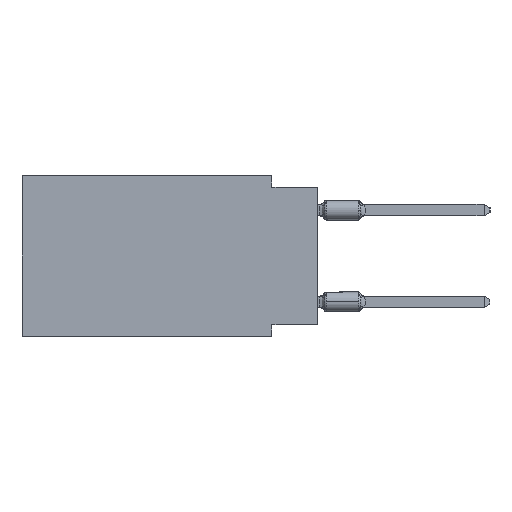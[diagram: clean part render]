
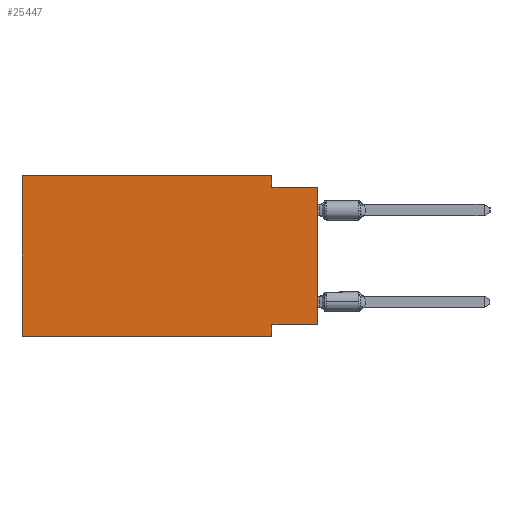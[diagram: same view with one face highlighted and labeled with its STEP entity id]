
A CAD part, left-side view. The second image highlights one B-rep face of the part: STEP entity #25447.
In plain terms, the highlighted planar face has unit normal (-1, 0, 0).
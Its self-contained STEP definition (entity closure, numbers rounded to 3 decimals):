
#44 = ORIENTED_EDGE ( 'NONE', *, *, #25093, .F. ) ;
#259 = LINE ( 'NONE', #33148, #37497 ) ;
#1192 = CARTESIAN_POINT ( 'NONE',  ( 0., 16.383, 0. ) ) ;
#1637 = VERTEX_POINT ( 'NONE', #36387 ) ;
#1899 = ORIENTED_EDGE ( 'NONE', *, *, #34662, .F. ) ;
#2124 = VERTEX_POINT ( 'NONE', #25669 ) ;
#2669 = ORIENTED_EDGE ( 'NONE', *, *, #28378, .F. ) ;
#2726 = VECTOR ( 'NONE', #9663, 1000. ) ;
#3540 = EDGE_CURVE ( 'NONE', #17082, #28157, #30162, .T. ) ;
#4827 = CARTESIAN_POINT ( 'NONE',  ( 0., 0., -8.255 ) ) ;
#5383 = VECTOR ( 'NONE', #29229, 1000. ) ;
#6342 = CARTESIAN_POINT ( 'NONE',  ( 0., 16.383, -8.89 ) ) ;
#7986 = DIRECTION ( 'NONE',  ( 0., 0., 1. ) ) ;
#9663 = DIRECTION ( 'NONE',  ( 0., -1., 0. ) ) ;
#9756 = ORIENTED_EDGE ( 'NONE', *, *, #12859, .F. ) ;
#10096 = CARTESIAN_POINT ( 'NONE',  ( 0., 0., -0.635 ) ) ;
#10932 = CARTESIAN_POINT ( 'NONE',  ( 0., 0., 0. ) ) ;
#10944 = VECTOR ( 'NONE', #24261, 1000. ) ;
#11020 = VERTEX_POINT ( 'NONE', #4827 ) ;
#12067 = LINE ( 'NONE', #21149, #21219 ) ;
#12614 = LINE ( 'NONE', #24622, #2726 ) ;
#12859 = EDGE_CURVE ( 'NONE', #11020, #26576, #22735, .T. ) ;
#13801 = VECTOR ( 'NONE', #31542, 1000. ) ;
#14263 = EDGE_CURVE ( 'NONE', #26576, #28157, #259, .T. ) ;
#16098 = PLANE ( 'NONE',  #33561 ) ;
#16342 = LINE ( 'NONE', #1192, #35155 ) ;
#16647 = EDGE_CURVE ( 'NONE', #11020, #26169, #37870, .T. ) ;
#17082 = VERTEX_POINT ( 'NONE', #27982 ) ;
#17401 = CARTESIAN_POINT ( 'NONE',  ( 0., 0., -8.255 ) ) ;
#19551 = LINE ( 'NONE', #10096, #13801 ) ;
#21149 = CARTESIAN_POINT ( 'NONE',  ( 0., 2.54, 0. ) ) ;
#21219 = VECTOR ( 'NONE', #27449, 1000. ) ;
#21431 = ORIENTED_EDGE ( 'NONE', *, *, #31875, .F. ) ;
#22735 = LINE ( 'NONE', #17401, #5383 ) ;
#24261 = DIRECTION ( 'NONE',  ( 0., -1., 0. ) ) ;
#24622 = CARTESIAN_POINT ( 'NONE',  ( 0., 16.383, 0. ) ) ;
#24906 = ORIENTED_EDGE ( 'NONE', *, *, #16647, .T. ) ;
#25093 = EDGE_CURVE ( 'NONE', #28184, #1637, #12614, .T. ) ;
#25159 = DIRECTION ( 'NONE',  ( 1., 0., 0. ) ) ;
#25247 = EDGE_LOOP ( 'NONE', ( #24906, #1899, #2669, #44, #21431, #28178, #38400, #9756 ) ) ;
#25447 = ADVANCED_FACE ( 'NONE', ( #36555 ), #16098, .F. ) ;
#25669 = CARTESIAN_POINT ( 'NONE',  ( 0., 2.54, -0.635 ) ) ;
#26169 = VERTEX_POINT ( 'NONE', #37380 ) ;
#26576 = VERTEX_POINT ( 'NONE', #27744 ) ;
#27449 = DIRECTION ( 'NONE',  ( 0., 0., -1. ) ) ;
#27744 = CARTESIAN_POINT ( 'NONE',  ( 0., 2.54, -8.255 ) ) ;
#27982 = CARTESIAN_POINT ( 'NONE',  ( 0., 16.383, -8.89 ) ) ;
#28129 = CARTESIAN_POINT ( 'NONE',  ( 0., 16.383, 0. ) ) ;
#28157 = VERTEX_POINT ( 'NONE', #35104 ) ;
#28178 = ORIENTED_EDGE ( 'NONE', *, *, #3540, .T. ) ;
#28184 = VERTEX_POINT ( 'NONE', #34911 ) ;
#28378 = EDGE_CURVE ( 'NONE', #1637, #2124, #12067, .T. ) ;
#29229 = DIRECTION ( 'NONE',  ( 0., 1., 0. ) ) ;
#30162 = LINE ( 'NONE', #6342, #10944 ) ;
#30912 = VECTOR ( 'NONE', #7986, 1000. ) ;
#31542 = DIRECTION ( 'NONE',  ( 0., -1., 0. ) ) ;
#31875 = EDGE_CURVE ( 'NONE', #17082, #28184, #16342, .T. ) ;
#33148 = CARTESIAN_POINT ( 'NONE',  ( 0., 2.54, -8.89 ) ) ;
#33561 = AXIS2_PLACEMENT_3D ( 'NONE', #28129, #25159, #37121 ) ;
#34052 = DIRECTION ( 'NONE',  ( 0., 0., 1. ) ) ;
#34662 = EDGE_CURVE ( 'NONE', #2124, #26169, #19551, .T. ) ;
#34911 = CARTESIAN_POINT ( 'NONE',  ( 0., 16.383, 0. ) ) ;
#35104 = CARTESIAN_POINT ( 'NONE',  ( 0., 2.54, -8.89 ) ) ;
#35155 = VECTOR ( 'NONE', #34052, 1000. ) ;
#36081 = DIRECTION ( 'NONE',  ( 0., 0., -1. ) ) ;
#36387 = CARTESIAN_POINT ( 'NONE',  ( 0., 2.54, 0. ) ) ;
#36555 = FACE_OUTER_BOUND ( 'NONE', #25247, .T. ) ;
#37121 = DIRECTION ( 'NONE',  ( 0., 0., -1. ) ) ;
#37380 = CARTESIAN_POINT ( 'NONE',  ( 0., 0., -0.635 ) ) ;
#37497 = VECTOR ( 'NONE', #36081, 1000. ) ;
#37870 = LINE ( 'NONE', #10932, #30912 ) ;
#38400 = ORIENTED_EDGE ( 'NONE', *, *, #14263, .F. ) ;
